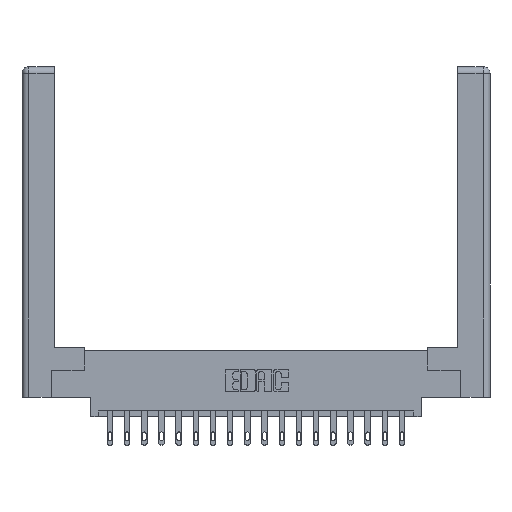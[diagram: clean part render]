
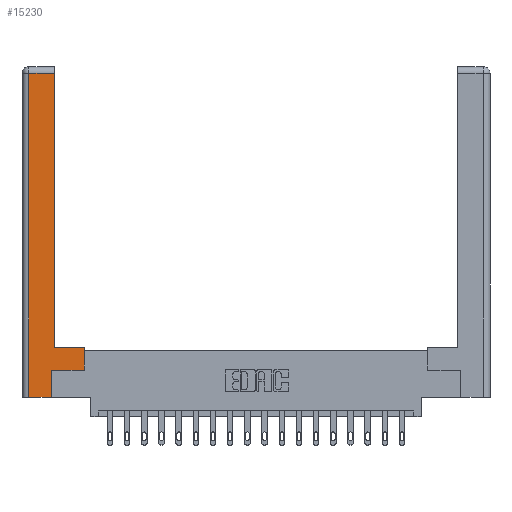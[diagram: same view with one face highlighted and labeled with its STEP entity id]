
A CAD part, top view. The second image highlights one B-rep face of the part: STEP entity #15230.
In plain terms, the highlighted planar face has unit normal (0, 0, 1).
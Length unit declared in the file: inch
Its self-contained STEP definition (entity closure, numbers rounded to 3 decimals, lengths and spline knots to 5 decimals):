
#1304 = VERTEX_POINT ( 'NONE', #8717 ) ;
#1598 = VERTEX_POINT ( 'NONE', #12322 ) ;
#1610 = CARTESIAN_POINT ( 'NONE',  ( 0.0615, 0., 0. ) ) ;
#1767 = VECTOR ( 'NONE', #14702, 39.37008 ) ;
#2296 = DIRECTION ( 'NONE',  ( -1., 0., 0. ) ) ;
#2473 = LINE ( 'NONE', #17589, #6038 ) ;
#2609 = EDGE_CURVE ( 'NONE', #1598, #19221, #2473, .T. ) ;
#2841 = DIRECTION ( 'NONE',  ( 0., 1., 0. ) ) ;
#3312 = CARTESIAN_POINT ( 'NONE',  ( 0.295, 2.94, 0. ) ) ;
#3536 = ORIENTED_EDGE ( 'NONE', *, *, #5524, .T. ) ;
#3876 = VECTOR ( 'NONE', #4839, 39.37008 ) ;
#4051 = ORIENTED_EDGE ( 'NONE', *, *, #4068, .T. ) ;
#4068 = EDGE_CURVE ( 'NONE', #19221, #16763, #11202, .T. ) ;
#4450 = ORIENTED_EDGE ( 'NONE', *, *, #2609, .T. ) ;
#4839 = DIRECTION ( 'NONE',  ( -1., 0., 0. ) ) ;
#4873 = LINE ( 'NONE', #6261, #8647 ) ;
#5524 = EDGE_CURVE ( 'NONE', #13599, #1304, #6482, .T. ) ;
#5635 = CARTESIAN_POINT ( 'NONE',  ( 0.565, 0.45, 0. ) ) ;
#5764 = CARTESIAN_POINT ( 'NONE',  ( 0.265, 0.245, 0. ) ) ;
#5807 = ORIENTED_EDGE ( 'NONE', *, *, #17878, .T. ) ;
#6038 = VECTOR ( 'NONE', #6823, 39.37008 ) ;
#6261 = CARTESIAN_POINT ( 'NONE',  ( 0.295, 0.45, 0. ) ) ;
#6482 = LINE ( 'NONE', #8005, #3876 ) ;
#6680 = LINE ( 'NONE', #9561, #18600 ) ;
#6823 = DIRECTION ( 'NONE',  ( 1., 0., 0. ) ) ;
#7015 = DIRECTION ( 'NONE',  ( 0., 0., -1. ) ) ;
#7841 = LINE ( 'NONE', #5635, #16657 ) ;
#8005 = CARTESIAN_POINT ( 'NONE',  ( 0.0615, 2.94, 0. ) ) ;
#8446 = LINE ( 'NONE', #8916, #1767 ) ;
#8509 = PLANE ( 'NONE',  #12702 ) ;
#8647 = VECTOR ( 'NONE', #13929, 39.37008 ) ;
#8717 = CARTESIAN_POINT ( 'NONE',  ( 0.0615, 2.94, 0. ) ) ;
#8916 = CARTESIAN_POINT ( 'NONE',  ( 0.295, 3., 0. ) ) ;
#9241 = EDGE_LOOP ( 'NONE', ( #16094, #3536, #9560, #4450, #4051, #5807, #11817, #14983 ) ) ;
#9560 = ORIENTED_EDGE ( 'NONE', *, *, #16704, .T. ) ;
#9561 = CARTESIAN_POINT ( 'NONE',  ( 0.565, 0.245, 0. ) ) ;
#9898 = VERTEX_POINT ( 'NONE', #11236 ) ;
#9952 = CARTESIAN_POINT ( 'NONE',  ( 0., 0., 0. ) ) ;
#9989 = VERTEX_POINT ( 'NONE', #13210 ) ;
#10014 = LINE ( 'NONE', #1610, #11915 ) ;
#11022 = FACE_OUTER_BOUND ( 'NONE', #9241, .T. ) ;
#11202 = LINE ( 'NONE', #5764, #12907 ) ;
#11236 = CARTESIAN_POINT ( 'NONE',  ( 0.565, 0.45, 0. ) ) ;
#11655 = EDGE_CURVE ( 'NONE', #9989, #9898, #7841, .T. ) ;
#11801 = DIRECTION ( 'NONE',  ( 0., 1., 0. ) ) ;
#11817 = ORIENTED_EDGE ( 'NONE', *, *, #11655, .T. ) ;
#11915 = VECTOR ( 'NONE', #12268, 39.37008 ) ;
#12268 = DIRECTION ( 'NONE',  ( 0., -1., 0. ) ) ;
#12322 = CARTESIAN_POINT ( 'NONE',  ( 0.0615, 0., 0. ) ) ;
#12702 = AXIS2_PLACEMENT_3D ( 'NONE', #9952, #7015, #2296 ) ;
#12907 = VECTOR ( 'NONE', #2841, 39.37008 ) ;
#13210 = CARTESIAN_POINT ( 'NONE',  ( 0.565, 0.245, 0. ) ) ;
#13599 = VERTEX_POINT ( 'NONE', #3312 ) ;
#13649 = DIRECTION ( 'NONE',  ( 1., 0., 0. ) ) ;
#13929 = DIRECTION ( 'NONE',  ( -1., 0., 0. ) ) ;
#14702 = DIRECTION ( 'NONE',  ( 0., 1., 0. ) ) ;
#14983 = ORIENTED_EDGE ( 'NONE', *, *, #15435, .T. ) ;
#15230 = ADVANCED_FACE ( 'NONE', ( #11022 ), #8509, .F. ) ;
#15435 = EDGE_CURVE ( 'NONE', #9898, #17330, #4873, .T. ) ;
#16094 = ORIENTED_EDGE ( 'NONE', *, *, #16907, .T. ) ;
#16657 = VECTOR ( 'NONE', #11801, 39.37008 ) ;
#16704 = EDGE_CURVE ( 'NONE', #1304, #1598, #10014, .T. ) ;
#16763 = VERTEX_POINT ( 'NONE', #19237 ) ;
#16907 = EDGE_CURVE ( 'NONE', #17330, #13599, #8446, .T. ) ;
#16931 = CARTESIAN_POINT ( 'NONE',  ( 0.295, 0.45, 0. ) ) ;
#17330 = VERTEX_POINT ( 'NONE', #16931 ) ;
#17589 = CARTESIAN_POINT ( 'NONE',  ( 0.265, 0., 0. ) ) ;
#17878 = EDGE_CURVE ( 'NONE', #16763, #9989, #6680, .T. ) ;
#18600 = VECTOR ( 'NONE', #13649, 39.37008 ) ;
#19221 = VERTEX_POINT ( 'NONE', #19347 ) ;
#19237 = CARTESIAN_POINT ( 'NONE',  ( 0.265, 0.245, 0. ) ) ;
#19347 = CARTESIAN_POINT ( 'NONE',  ( 0.265, 0., 0. ) ) ;
